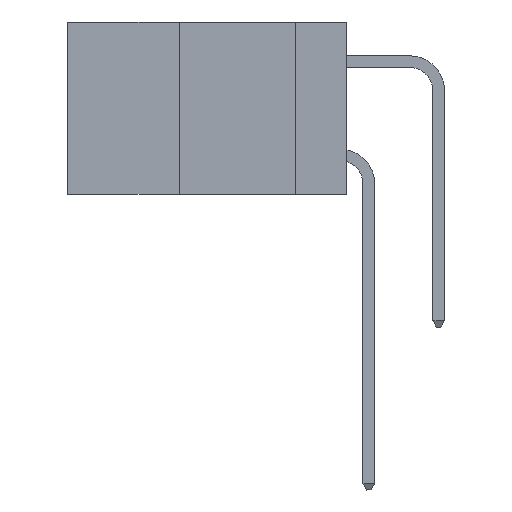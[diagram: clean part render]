
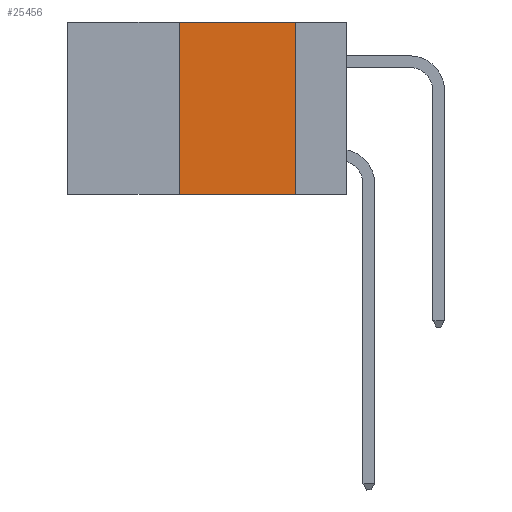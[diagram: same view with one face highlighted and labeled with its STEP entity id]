
A CAD part, left-side view. The second image highlights one B-rep face of the part: STEP entity #25456.
In plain terms, the highlighted planar face has unit normal (-1, 0, 0).
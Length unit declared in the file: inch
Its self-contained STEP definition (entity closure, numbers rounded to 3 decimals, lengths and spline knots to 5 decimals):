
#429 = EDGE_CURVE ( 'NONE', #11004, #23655, #16695, .T. ) ;
#4028 = DIRECTION ( 'NONE',  ( 0., 0., 1. ) ) ;
#4511 = LINE ( 'NONE', #18921, #6009 ) ;
#5310 = CARTESIAN_POINT ( 'NONE',  ( 0., 0.36, 0. ) ) ;
#6009 = VECTOR ( 'NONE', #18041, 39.37008 ) ;
#6184 = LINE ( 'NONE', #8455, #6584 ) ;
#6584 = VECTOR ( 'NONE', #17738, 39.37008 ) ;
#7105 = ORIENTED_EDGE ( 'NONE', *, *, #429, .F. ) ;
#7390 = CARTESIAN_POINT ( 'NONE',  ( 0., 0.11, 0. ) ) ;
#7543 = DIRECTION ( 'NONE',  ( 0., 0., -1. ) ) ;
#7568 = CARTESIAN_POINT ( 'NONE',  ( 0., 0.36, -0.37 ) ) ;
#8455 = CARTESIAN_POINT ( 'NONE',  ( 0., 0.6, -0.37 ) ) ;
#10747 = PLANE ( 'NONE',  #22040 ) ;
#11004 = VERTEX_POINT ( 'NONE', #7390 ) ;
#13044 = DIRECTION ( 'NONE',  ( 0., 0., -1. ) ) ;
#15895 = ORIENTED_EDGE ( 'NONE', *, *, #26821, .T. ) ;
#16660 = ORIENTED_EDGE ( 'NONE', *, *, #26008, .F. ) ;
#16695 = LINE ( 'NONE', #18969, #22740 ) ;
#17055 = EDGE_LOOP ( 'NONE', ( #7105, #18855, #16660, #15895 ) ) ;
#17738 = DIRECTION ( 'NONE',  ( 0., -1., 0. ) ) ;
#18041 = DIRECTION ( 'NONE',  ( 0., -1., 0. ) ) ;
#18821 = VERTEX_POINT ( 'NONE', #7568 ) ;
#18855 = ORIENTED_EDGE ( 'NONE', *, *, #24361, .F. ) ;
#18921 = CARTESIAN_POINT ( 'NONE',  ( 0., 0.6, 0. ) ) ;
#18969 = CARTESIAN_POINT ( 'NONE',  ( 0., 0.11, 0. ) ) ;
#19639 = VECTOR ( 'NONE', #4028, 39.37008 ) ;
#20880 = CARTESIAN_POINT ( 'NONE',  ( 0., 0.36, 0. ) ) ;
#22040 = AXIS2_PLACEMENT_3D ( 'NONE', #26825, #26675, #13044 ) ;
#22282 = FACE_OUTER_BOUND ( 'NONE', #17055, .T. ) ;
#22314 = CARTESIAN_POINT ( 'NONE',  ( 0., 0.11, -0.37 ) ) ;
#22740 = VECTOR ( 'NONE', #7543, 39.37008 ) ;
#23655 = VERTEX_POINT ( 'NONE', #22314 ) ;
#24361 = EDGE_CURVE ( 'NONE', #27522, #11004, #4511, .T. ) ;
#24820 = LINE ( 'NONE', #20880, #19639 ) ;
#25456 = ADVANCED_FACE ( 'NONE', ( #22282 ), #10747, .F. ) ;
#26008 = EDGE_CURVE ( 'NONE', #18821, #27522, #24820, .T. ) ;
#26675 = DIRECTION ( 'NONE',  ( 1., 0., 0. ) ) ;
#26821 = EDGE_CURVE ( 'NONE', #18821, #23655, #6184, .T. ) ;
#26825 = CARTESIAN_POINT ( 'NONE',  ( 0., 0.6, 0. ) ) ;
#27522 = VERTEX_POINT ( 'NONE', #5310 ) ;
